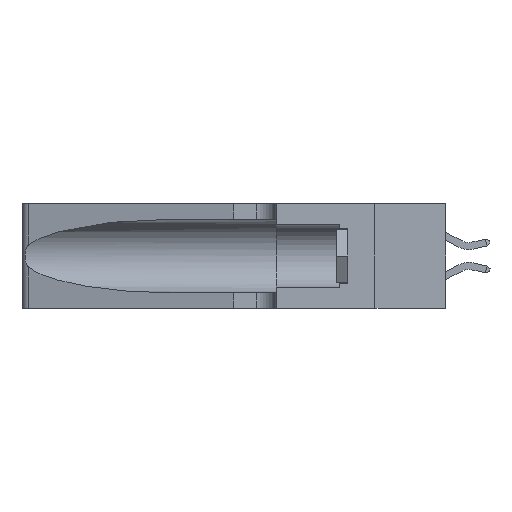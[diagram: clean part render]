
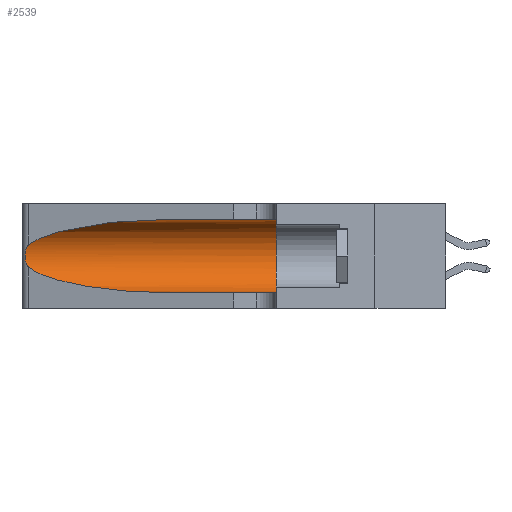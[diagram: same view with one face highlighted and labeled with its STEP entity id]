
A CAD part, left-side view. The second image highlights one B-rep face of the part: STEP entity #2539.
In plain terms, the highlighted cylindrical face has radius 3.308 mm (diameter 6.617 mm), a partial arc.
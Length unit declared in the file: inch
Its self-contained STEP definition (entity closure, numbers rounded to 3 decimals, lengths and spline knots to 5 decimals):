
#298 = ORIENTED_EDGE ( 'NONE', *, *, #18057, .F. ) ;
#846 = CARTESIAN_POINT ( 'NONE',  ( 0.25787, 1.23484, 0.2124 ) ) ;
#2032 = CARTESIAN_POINT ( 'NONE',  ( 0.25487, 1.22718, 0.22369 ) ) ;
#2539 = ADVANCED_FACE ( 'NONE', ( #22019 ), #5644, .F. ) ;
#3040 = VECTOR ( 'NONE', #24578, 39.37008 ) ;
#3222 = CARTESIAN_POINT ( 'NONE',  ( 0.26017, 1.23833, 0.17102 ) ) ;
#3415 = CARTESIAN_POINT ( 'NONE',  ( 0.25854, 1.2359, 0.20912 ) ) ;
#3845 = CARTESIAN_POINT ( 'NONE',  ( 0.1305, 0.72297, 0.31525 ) ) ;
#5407 = CARTESIAN_POINT ( 'NONE',  ( 0.25856, 1.23593, 0.16098 ) ) ;
#5644 = CYLINDRICAL_SURFACE ( 'NONE', #21432, 0.13025 ) ;
#5708 = ORIENTED_EDGE ( 'NONE', *, *, #6594, .T. ) ;
#6087 = LINE ( 'NONE', #9317, #3040 ) ;
#6136 = CARTESIAN_POINT ( 'NONE',  ( 0.1305, 0.35, 0.31525 ) ) ;
#6200 = VECTOR ( 'NONE', #26308, 39.37008 ) ;
#6476 = CARTESIAN_POINT ( 'NONE',  ( 0.25487, 1.22718, 0.22369 ) ) ;
#6594 = EDGE_CURVE ( 'NONE', #14039, #24856, #6087, .T. ) ;
#6670 = CARTESIAN_POINT ( 'NONE',  ( 0.1305, 0.72297, 0.31525 ) ) ;
#7733 = EDGE_CURVE ( 'NONE', #26621, #14039, #16895, .T. ) ;
#7752 = ORIENTED_EDGE ( 'NONE', *, *, #11373, .T. ) ;
#8154 = VERTEX_POINT ( 'NONE', #3845 ) ;
#9062 = CARTESIAN_POINT ( 'NONE',  ( 0.1305, 1.61858, 0.31525 ) ) ;
#9317 = CARTESIAN_POINT ( 'NONE',  ( 0.1305, 1.61858, 0.05475 ) ) ;
#9652 = CARTESIAN_POINT ( 'NONE',  ( 0.25555, 1.22994, 0.2215 ) ) ;
#9750 = VERTEX_POINT ( 'NONE', #6136 ) ;
#10516 = VERTEX_POINT ( 'NONE', #6476 ) ;
#10902 = CARTESIAN_POINT ( 'NONE',  ( 0.1305, 0.35, 0.05475 ) ) ;
#10986 = ORIENTED_EDGE ( 'NONE', *, *, #11764, .F. ) ;
#11373 = EDGE_CURVE ( 'NONE', #10516, #26621, #19881, .T. ) ;
#11478 = DIRECTION ( 'NONE',  ( 0., 0., 1. ) ) ;
#11693 = ORIENTED_EDGE ( 'NONE', *, *, #12418, .T. ) ;
#11764 = EDGE_CURVE ( 'NONE', #8154, #9750, #27641, .T. ) ;
#12418 = EDGE_CURVE ( 'NONE', #8154, #10516, #25786, .T. ) ;
#12557 = CARTESIAN_POINT ( 'NONE',  ( 0.2373, 1.15595, 0.08982 ) ) ;
#14039 = VERTEX_POINT ( 'NONE', #17372 ) ;
#14234 = CARTESIAN_POINT ( 'NONE',  ( 0.25639, 1.23186, 0.15144 ) ) ;
#15022 = EDGE_LOOP ( 'NONE', ( #11693, #7752, #21529, #5708, #298, #10986 ) ) ;
#16258 = CARTESIAN_POINT ( 'NONE',  ( 0.26075, 1.23896, 0.178 ) ) ;
#16352 = CARTESIAN_POINT ( 'NONE',  ( 0.25487, 1.22718, 0.14631 ) ) ;
#16409 = CIRCLE ( 'NONE', #23814, 0.13025 ) ;
#16895 =( BOUNDED_CURVE ( )  B_SPLINE_CURVE ( 3, ( #19167, #12557, #25437, #21186 ),
 .UNSPECIFIED., .F., .F. ) 
 B_SPLINE_CURVE_WITH_KNOTS ( ( 4, 4 ),
 ( 3.44316, 4.71239 ),
 .UNSPECIFIED. ) 
 CURVE ( )  GEOMETRIC_REPRESENTATION_ITEM ( )  RATIONAL_B_SPLINE_CURVE ( ( 1., 0.87, 0.87, 1. ) ) 
 REPRESENTATION_ITEM ( '' )  );
#17372 = CARTESIAN_POINT ( 'NONE',  ( 0.1305, 0.72297, 0.05475 ) ) ;
#18057 = EDGE_CURVE ( 'NONE', #9750, #24856, #16409, .T. ) ;
#18325 = DIRECTION ( 'NONE',  ( 0., 0., -1. ) ) ;
#18558 = CARTESIAN_POINT ( 'NONE',  ( 0.25639, 1.23184, 0.21858 ) ) ;
#18711 = CARTESIAN_POINT ( 'NONE',  ( 0.1305, 1.61858, 0.185 ) ) ;
#19167 = CARTESIAN_POINT ( 'NONE',  ( 0.25487, 1.22718, 0.14631 ) ) ;
#19375 = CARTESIAN_POINT ( 'NONE',  ( 0.18966, 0.96281, 0.31525 ) ) ;
#19881 = B_SPLINE_CURVE_WITH_KNOTS ( 'NONE', 3,
 ( #27210, #9652, #18558, #846, #3415, #24920, #27120, #16258, #3222, #5407, #20670, #14234, #22836, #16352 ),
 .UNSPECIFIED., .F., .F.,
 ( 4, 2, 2, 2, 2, 2, 4 ),
 ( 0., 0.00027, 0.00053, 0.00107, 0.0016, 0.00187, 0.00214 ),
 .UNSPECIFIED. ) ;
#20285 = CARTESIAN_POINT ( 'NONE',  ( 0.1305, 0.35, 0.185 ) ) ;
#20670 = CARTESIAN_POINT ( 'NONE',  ( 0.25789, 1.23486, 0.15765 ) ) ;
#21186 = CARTESIAN_POINT ( 'NONE',  ( 0.1305, 0.72297, 0.05475 ) ) ;
#21432 = AXIS2_PLACEMENT_3D ( 'NONE', #18711, #27171, #18325 ) ;
#21529 = ORIENTED_EDGE ( 'NONE', *, *, #7733, .T. ) ;
#21646 = CARTESIAN_POINT ( 'NONE',  ( 0.2373, 1.15595, 0.28018 ) ) ;
#22019 = FACE_OUTER_BOUND ( 'NONE', #15022, .T. ) ;
#22836 = CARTESIAN_POINT ( 'NONE',  ( 0.25555, 1.22993, 0.14849 ) ) ;
#23814 = AXIS2_PLACEMENT_3D ( 'NONE', #20285, #24366, #11478 ) ;
#24366 = DIRECTION ( 'NONE',  ( 0., 1., 0. ) ) ;
#24578 = DIRECTION ( 'NONE',  ( 0., -1., 0. ) ) ;
#24856 = VERTEX_POINT ( 'NONE', #10902 ) ;
#24920 = CARTESIAN_POINT ( 'NONE',  ( 0.26018, 1.23835, 0.19895 ) ) ;
#25437 = CARTESIAN_POINT ( 'NONE',  ( 0.18966, 0.96281, 0.05475 ) ) ;
#25551 = CARTESIAN_POINT ( 'NONE',  ( 0.25487, 1.22718, 0.14631 ) ) ;
#25786 =( BOUNDED_CURVE ( )  B_SPLINE_CURVE ( 3, ( #6670, #19375, #21646, #2032 ),
 .UNSPECIFIED., .F., .F. ) 
 B_SPLINE_CURVE_WITH_KNOTS ( ( 4, 4 ),
 ( 1.5708, 2.84003 ),
 .UNSPECIFIED. ) 
 CURVE ( )  GEOMETRIC_REPRESENTATION_ITEM ( )  RATIONAL_B_SPLINE_CURVE ( ( 1., 0.87, 0.87, 1. ) ) 
 REPRESENTATION_ITEM ( '' )  );
#26308 = DIRECTION ( 'NONE',  ( 0., -1., 0. ) ) ;
#26621 = VERTEX_POINT ( 'NONE', #25551 ) ;
#27120 = CARTESIAN_POINT ( 'NONE',  ( 0.26075, 1.23896, 0.19203 ) ) ;
#27171 = DIRECTION ( 'NONE',  ( 0., -1., 0. ) ) ;
#27210 = CARTESIAN_POINT ( 'NONE',  ( 0.25487, 1.22718, 0.22369 ) ) ;
#27641 = LINE ( 'NONE', #9062, #6200 ) ;
